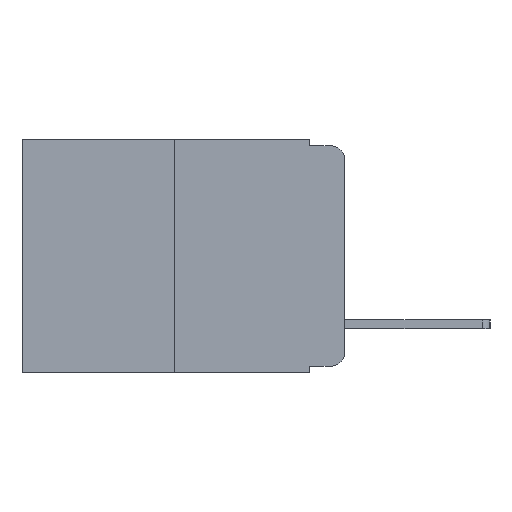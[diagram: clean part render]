
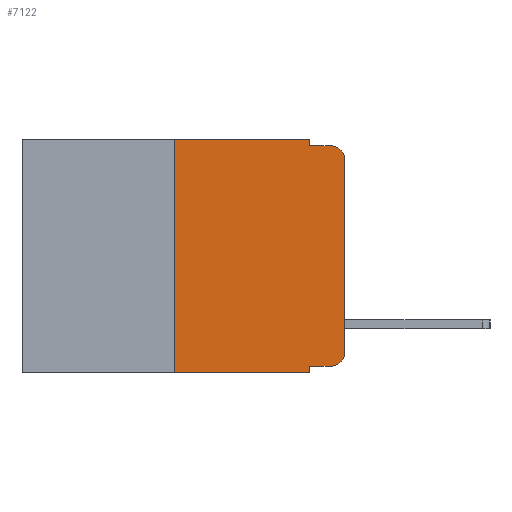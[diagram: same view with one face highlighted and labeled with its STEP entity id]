
A CAD part, left-side view. The second image highlights one B-rep face of the part: STEP entity #7122.
In plain terms, the highlighted planar face has unit normal (-1, 0, 0).
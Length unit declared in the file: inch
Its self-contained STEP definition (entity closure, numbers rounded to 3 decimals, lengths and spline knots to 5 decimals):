
#10 = EDGE_CURVE ( 'NONE', #9429, #17391, #9798, .T. ) ;
#525 = VERTEX_POINT ( 'NONE', #6698 ) ;
#565 = DIRECTION ( 'NONE',  ( -1., 0., 0. ) ) ;
#657 = CARTESIAN_POINT ( 'NONE',  ( 0., 0.473, 0. ) ) ;
#876 = CARTESIAN_POINT ( 'NONE',  ( 0., 0.051, -0.01 ) ) ;
#1530 = CARTESIAN_POINT ( 'NONE',  ( 0., 0.25, 0. ) ) ;
#1700 = DIRECTION ( 'NONE',  ( 0., 0., -1. ) ) ;
#1849 = CARTESIAN_POINT ( 'NONE',  ( 0., 0.051, -0.333 ) ) ;
#2275 = CARTESIAN_POINT ( 'NONE',  ( 0., 0.051, -0.333 ) ) ;
#2507 = CARTESIAN_POINT ( 'NONE',  ( 0., 0.051, -0.01 ) ) ;
#2598 = VECTOR ( 'NONE', #14580, 39.37008 ) ;
#3034 = EDGE_CURVE ( 'NONE', #14222, #4103, #10891, .T. ) ;
#3146 = VECTOR ( 'NONE', #4450, 39.37008 ) ;
#3239 = CARTESIAN_POINT ( 'NONE',  ( 0., 0.25, -0.343 ) ) ;
#3291 = EDGE_CURVE ( 'NONE', #14222, #17391, #17698, .T. ) ;
#3376 = DIRECTION ( 'NONE',  ( -1., 0., 0. ) ) ;
#3972 = CARTESIAN_POINT ( 'NONE',  ( 0., 0., -0.03 ) ) ;
#4031 = EDGE_CURVE ( 'NONE', #4214, #12737, #5666, .T. ) ;
#4103 = VERTEX_POINT ( 'NONE', #10580 ) ;
#4214 = VERTEX_POINT ( 'NONE', #17816 ) ;
#4362 = CARTESIAN_POINT ( 'NONE',  ( 0., 0.051, -0.343 ) ) ;
#4450 = DIRECTION ( 'NONE',  ( 0., 0., 1. ) ) ;
#4561 = CARTESIAN_POINT ( 'NONE',  ( 0., 0.473, 0. ) ) ;
#4890 = DIRECTION ( 'NONE',  ( 0., 0., 1. ) ) ;
#4952 = VERTEX_POINT ( 'NONE', #18087 ) ;
#5024 = EDGE_CURVE ( 'NONE', #12737, #525, #18256, .T. ) ;
#5666 = LINE ( 'NONE', #10456, #9527 ) ;
#5944 = VECTOR ( 'NONE', #13223, 39.37008 ) ;
#6013 = EDGE_CURVE ( 'NONE', #18043, #525, #9239, .T. ) ;
#6562 = DIRECTION ( 'NONE',  ( 0., -1., 0. ) ) ;
#6629 = DIRECTION ( 'NONE',  ( 1., 0., 0. ) ) ;
#6698 = CARTESIAN_POINT ( 'NONE',  ( 0., 0.02, -0.01 ) ) ;
#6992 = VECTOR ( 'NONE', #11230, 39.37008 ) ;
#6998 = EDGE_CURVE ( 'NONE', #18330, #18043, #14497, .T. ) ;
#7122 = ADVANCED_FACE ( 'NONE', ( #9425 ), #15145, .F. ) ;
#7493 = AXIS2_PLACEMENT_3D ( 'NONE', #9396, #565, #10821 ) ;
#7504 = EDGE_CURVE ( 'NONE', #4103, #4214, #17383, .T. ) ;
#8708 = AXIS2_PLACEMENT_3D ( 'NONE', #657, #6629, #16556 ) ;
#8850 = LINE ( 'NONE', #2275, #15921 ) ;
#9239 = CIRCLE ( 'NONE', #15801, 0.02 ) ;
#9396 = CARTESIAN_POINT ( 'NONE',  ( 0., 0.02, -0.313 ) ) ;
#9425 = FACE_OUTER_BOUND ( 'NONE', #9852, .T. ) ;
#9429 = VERTEX_POINT ( 'NONE', #1849 ) ;
#9527 = VECTOR ( 'NONE', #1700, 39.37008 ) ;
#9798 = LINE ( 'NONE', #17021, #5944 ) ;
#9852 = EDGE_LOOP ( 'NONE', ( #15520, #14868, #14817, #14939, #14780, #14800, #15465, #15498, #15396, #15431 ) ) ;
#10456 = CARTESIAN_POINT ( 'NONE',  ( 0., 0.051, 0. ) ) ;
#10580 = CARTESIAN_POINT ( 'NONE',  ( 0., 0.25, 0. ) ) ;
#10675 = VECTOR ( 'NONE', #6562, 39.37008 ) ;
#10761 = VECTOR ( 'NONE', #4890, 39.37008 ) ;
#10821 = DIRECTION ( 'NONE',  ( 0., 0., -1. ) ) ;
#10891 = LINE ( 'NONE', #1530, #3146 ) ;
#11230 = DIRECTION ( 'NONE',  ( 0., -1., 0. ) ) ;
#11792 = CIRCLE ( 'NONE', #7493, 0.02 ) ;
#12054 = CARTESIAN_POINT ( 'NONE',  ( 0., 0.02, -0.03 ) ) ;
#12471 = DIRECTION ( 'NONE',  ( 0., -1., 0. ) ) ;
#12737 = VERTEX_POINT ( 'NONE', #876 ) ;
#13223 = DIRECTION ( 'NONE',  ( 0., 0., -1. ) ) ;
#13462 = DIRECTION ( 'NONE',  ( 0., 0., -1. ) ) ;
#14222 = VERTEX_POINT ( 'NONE', #3239 ) ;
#14497 = LINE ( 'NONE', #14840, #10761 ) ;
#14580 = DIRECTION ( 'NONE',  ( 0., -1., 0. ) ) ;
#14693 = CARTESIAN_POINT ( 'NONE',  ( 0., 0., -0.313 ) ) ;
#14780 = ORIENTED_EDGE ( 'NONE', *, *, #7504, .F. ) ;
#14800 = ORIENTED_EDGE ( 'NONE', *, *, #3034, .F. ) ;
#14817 = ORIENTED_EDGE ( 'NONE', *, *, #5024, .F. ) ;
#14840 = CARTESIAN_POINT ( 'NONE',  ( 0., 0., 0. ) ) ;
#14868 = ORIENTED_EDGE ( 'NONE', *, *, #6013, .T. ) ;
#14939 = ORIENTED_EDGE ( 'NONE', *, *, #4031, .F. ) ;
#15145 = PLANE ( 'NONE',  #8708 ) ;
#15396 = ORIENTED_EDGE ( 'NONE', *, *, #17780, .T. ) ;
#15431 = ORIENTED_EDGE ( 'NONE', *, *, #15914, .T. ) ;
#15465 = ORIENTED_EDGE ( 'NONE', *, *, #3291, .T. ) ;
#15498 = ORIENTED_EDGE ( 'NONE', *, *, #10, .F. ) ;
#15520 = ORIENTED_EDGE ( 'NONE', *, *, #6998, .T. ) ;
#15801 = AXIS2_PLACEMENT_3D ( 'NONE', #12054, #3376, #13462 ) ;
#15914 = EDGE_CURVE ( 'NONE', #4952, #18330, #11792, .T. ) ;
#15921 = VECTOR ( 'NONE', #12471, 39.37008 ) ;
#16495 = CARTESIAN_POINT ( 'NONE',  ( 0., 0.473, -0.343 ) ) ;
#16556 = DIRECTION ( 'NONE',  ( 0., 0., -1. ) ) ;
#17021 = CARTESIAN_POINT ( 'NONE',  ( 0., 0.051, 0. ) ) ;
#17383 = LINE ( 'NONE', #4561, #2598 ) ;
#17391 = VERTEX_POINT ( 'NONE', #4362 ) ;
#17698 = LINE ( 'NONE', #16495, #10675 ) ;
#17780 = EDGE_CURVE ( 'NONE', #9429, #4952, #8850, .T. ) ;
#17816 = CARTESIAN_POINT ( 'NONE',  ( 0., 0.051, 0. ) ) ;
#18043 = VERTEX_POINT ( 'NONE', #3972 ) ;
#18087 = CARTESIAN_POINT ( 'NONE',  ( 0., 0.02, -0.333 ) ) ;
#18256 = LINE ( 'NONE', #2507, #6992 ) ;
#18330 = VERTEX_POINT ( 'NONE', #14693 ) ;
